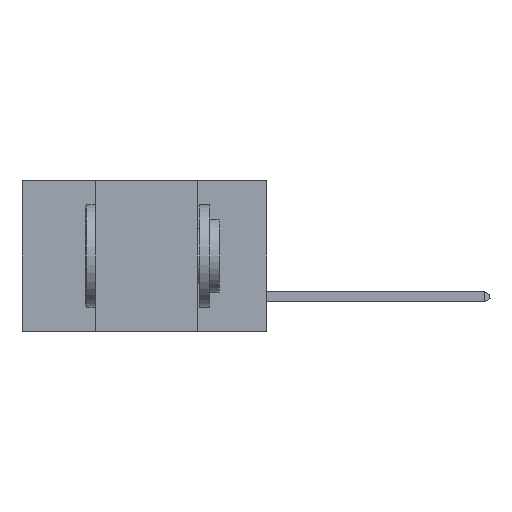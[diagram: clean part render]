
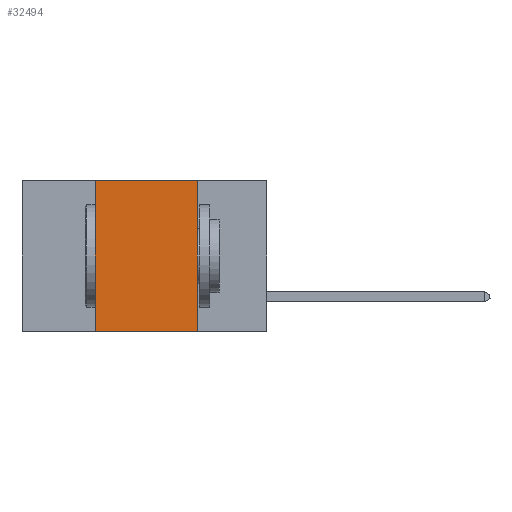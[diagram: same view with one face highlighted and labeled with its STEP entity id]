
A CAD part, left-side view. The second image highlights one B-rep face of the part: STEP entity #32494.
In plain terms, the highlighted planar face has unit normal (-1, 0, 0).
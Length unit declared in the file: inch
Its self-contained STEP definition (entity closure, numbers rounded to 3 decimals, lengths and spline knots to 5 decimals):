
#1047 = VECTOR ( 'NONE', #10481, 39.37008 ) ;
#1507 = DIRECTION ( 'NONE',  ( 0., 0., -1. ) ) ;
#2823 = DIRECTION ( 'NONE',  ( 0., -1., 0. ) ) ;
#4512 = LINE ( 'NONE', #14973, #12105 ) ;
#5657 = ORIENTED_EDGE ( 'NONE', *, *, #23812, .F. ) ;
#5929 = CARTESIAN_POINT ( 'NONE',  ( 0., 0.6, -0.37 ) ) ;
#6390 = VERTEX_POINT ( 'NONE', #30924 ) ;
#9700 = LINE ( 'NONE', #34193, #35276 ) ;
#10481 = DIRECTION ( 'NONE',  ( 0., 0., 1. ) ) ;
#10906 = AXIS2_PLACEMENT_3D ( 'NONE', #13947, #13540, #1507 ) ;
#11283 = LINE ( 'NONE', #5929, #25464 ) ;
#12105 = VECTOR ( 'NONE', #2823, 39.37008 ) ;
#12326 = DIRECTION ( 'NONE',  ( 0., -1., 0. ) ) ;
#12336 = CARTESIAN_POINT ( 'NONE',  ( 0., 0.17, -0.37 ) ) ;
#12569 = FACE_OUTER_BOUND ( 'NONE', #14218, .T. ) ;
#13540 = DIRECTION ( 'NONE',  ( 1., 0., 0. ) ) ;
#13947 = CARTESIAN_POINT ( 'NONE',  ( 0., 0.6, 0. ) ) ;
#14218 = EDGE_LOOP ( 'NONE', ( #18405, #35241, #5657, #29438 ) ) ;
#14973 = CARTESIAN_POINT ( 'NONE',  ( 0., 0.6, 0. ) ) ;
#18405 = ORIENTED_EDGE ( 'NONE', *, *, #32790, .F. ) ;
#22068 = EDGE_CURVE ( 'NONE', #6390, #29596, #4512, .T. ) ;
#22544 = CARTESIAN_POINT ( 'NONE',  ( 0., 0.42, 0. ) ) ;
#23812 = EDGE_CURVE ( 'NONE', #26511, #6390, #28504, .T. ) ;
#23983 = VERTEX_POINT ( 'NONE', #12336 ) ;
#25464 = VECTOR ( 'NONE', #12326, 39.37008 ) ;
#26511 = VERTEX_POINT ( 'NONE', #35648 ) ;
#27635 = DIRECTION ( 'NONE',  ( 0., 0., -1. ) ) ;
#28504 = LINE ( 'NONE', #22544, #1047 ) ;
#29438 = ORIENTED_EDGE ( 'NONE', *, *, #37605, .T. ) ;
#29596 = VERTEX_POINT ( 'NONE', #38604 ) ;
#30924 = CARTESIAN_POINT ( 'NONE',  ( 0., 0.42, 0. ) ) ;
#32494 = ADVANCED_FACE ( 'NONE', ( #12569 ), #34822, .F. ) ;
#32790 = EDGE_CURVE ( 'NONE', #29596, #23983, #9700, .T. ) ;
#34193 = CARTESIAN_POINT ( 'NONE',  ( 0., 0.17, 0. ) ) ;
#34822 = PLANE ( 'NONE',  #10906 ) ;
#35241 = ORIENTED_EDGE ( 'NONE', *, *, #22068, .F. ) ;
#35276 = VECTOR ( 'NONE', #27635, 39.37008 ) ;
#35648 = CARTESIAN_POINT ( 'NONE',  ( 0., 0.42, -0.37 ) ) ;
#37605 = EDGE_CURVE ( 'NONE', #26511, #23983, #11283, .T. ) ;
#38604 = CARTESIAN_POINT ( 'NONE',  ( 0., 0.17, 0. ) ) ;
